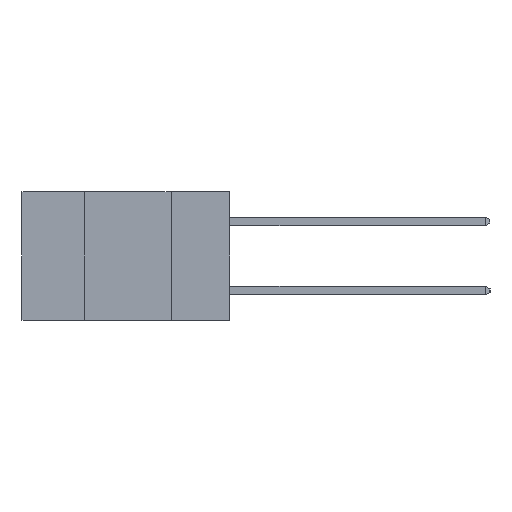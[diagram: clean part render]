
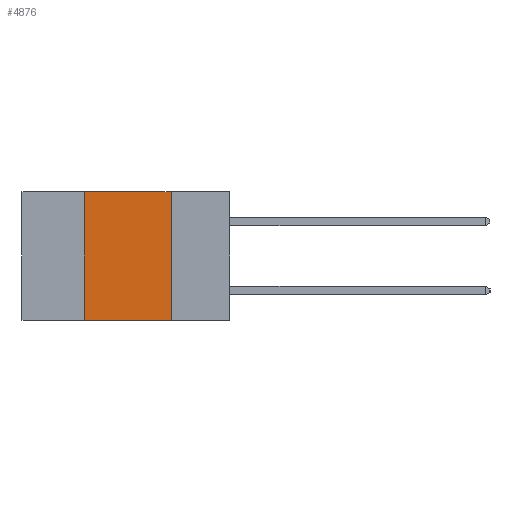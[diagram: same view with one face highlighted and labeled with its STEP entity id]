
A CAD part, left-side view. The second image highlights one B-rep face of the part: STEP entity #4876.
In plain terms, the highlighted planar face has unit normal (-1, 0, 0).
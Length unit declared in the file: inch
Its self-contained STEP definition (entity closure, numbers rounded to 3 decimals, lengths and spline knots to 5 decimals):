
#722 = CARTESIAN_POINT ( 'NONE',  ( 0., 0.42, -0.37 ) ) ;
#1152 = CARTESIAN_POINT ( 'NONE',  ( 0., 0.6, -0.37 ) ) ;
#1523 = DIRECTION ( 'NONE',  ( 0., 0., -1. ) ) ;
#1531 = DIRECTION ( 'NONE',  ( 1., 0., 0. ) ) ;
#1544 = PLANE ( 'NONE',  #8254 ) ;
#1670 = VECTOR ( 'NONE', #1958, 39.37008 ) ;
#1698 = CARTESIAN_POINT ( 'NONE',  ( 0., 0.6, 0. ) ) ;
#1792 = VERTEX_POINT ( 'NONE', #722 ) ;
#1958 = DIRECTION ( 'NONE',  ( 0., -1., 0. ) ) ;
#1990 = FACE_OUTER_BOUND ( 'NONE', #8584, .T. ) ;
#2232 = CARTESIAN_POINT ( 'NONE',  ( 0., 0.17, 0. ) ) ;
#2376 = CARTESIAN_POINT ( 'NONE',  ( 0., 0.42, 0. ) ) ;
#2930 = CARTESIAN_POINT ( 'NONE',  ( 0., 0.17, -0.37 ) ) ;
#3595 = VERTEX_POINT ( 'NONE', #6189 ) ;
#4093 = VECTOR ( 'NONE', #9835, 39.37008 ) ;
#4316 = EDGE_CURVE ( 'NONE', #1792, #7731, #8755, .T. ) ;
#4798 = ORIENTED_EDGE ( 'NONE', *, *, #7555, .F. ) ;
#4876 = ADVANCED_FACE ( 'NONE', ( #1990 ), #1544, .F. ) ;
#5833 = LINE ( 'NONE', #1152, #1670 ) ;
#5931 = CARTESIAN_POINT ( 'NONE',  ( 0., 0.6, 0. ) ) ;
#6189 = CARTESIAN_POINT ( 'NONE',  ( 0., 0.17, -0.37 ) ) ;
#6671 = VECTOR ( 'NONE', #8706, 39.37008 ) ;
#7419 = ORIENTED_EDGE ( 'NONE', *, *, #9309, .F. ) ;
#7555 = EDGE_CURVE ( 'NONE', #7612, #3595, #8453, .T. ) ;
#7612 = VERTEX_POINT ( 'NONE', #2232 ) ;
#7657 = DIRECTION ( 'NONE',  ( 0., 0., -1. ) ) ;
#7731 = VERTEX_POINT ( 'NONE', #2376 ) ;
#8040 = EDGE_CURVE ( 'NONE', #1792, #3595, #5833, .T. ) ;
#8254 = AXIS2_PLACEMENT_3D ( 'NONE', #1698, #1531, #1523 ) ;
#8453 = LINE ( 'NONE', #2930, #9972 ) ;
#8552 = LINE ( 'NONE', #5931, #4093 ) ;
#8584 = EDGE_LOOP ( 'NONE', ( #4798, #7419, #9504, #9763 ) ) ;
#8650 = CARTESIAN_POINT ( 'NONE',  ( 0., 0.42, -0.37 ) ) ;
#8706 = DIRECTION ( 'NONE',  ( 0., 0., 1. ) ) ;
#8755 = LINE ( 'NONE', #8650, #6671 ) ;
#9309 = EDGE_CURVE ( 'NONE', #7731, #7612, #8552, .T. ) ;
#9504 = ORIENTED_EDGE ( 'NONE', *, *, #4316, .F. ) ;
#9763 = ORIENTED_EDGE ( 'NONE', *, *, #8040, .T. ) ;
#9835 = DIRECTION ( 'NONE',  ( 0., -1., 0. ) ) ;
#9972 = VECTOR ( 'NONE', #7657, 39.37008 ) ;
